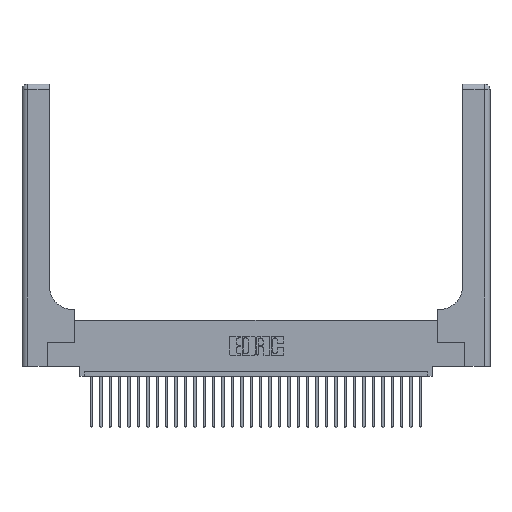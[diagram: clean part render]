
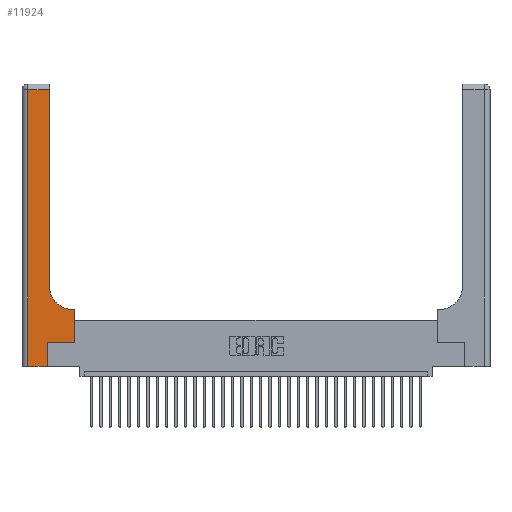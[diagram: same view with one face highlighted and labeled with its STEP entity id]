
A CAD part, top view. The second image highlights one B-rep face of the part: STEP entity #11924.
In plain terms, the highlighted planar face has unit normal (0, 0, 1).
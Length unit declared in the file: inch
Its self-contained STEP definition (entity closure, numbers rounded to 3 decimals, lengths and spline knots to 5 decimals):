
#829 = DIRECTION ( 'NONE',  ( 1., 0., 0. ) ) ;
#990 = EDGE_CURVE ( 'NONE', #28416, #30081, #33058, .T. ) ;
#1725 = VERTEX_POINT ( 'NONE', #17095 ) ;
#1779 = FACE_OUTER_BOUND ( 'NONE', #15088, .T. ) ;
#1963 = CARTESIAN_POINT ( 'NONE',  ( 0.06, 0., 0.37 ) ) ;
#2214 = CARTESIAN_POINT ( 'NONE',  ( 0.5415, 0.6, 0.37 ) ) ;
#3180 = DIRECTION ( 'NONE',  ( 0., 0., -1. ) ) ;
#3660 = EDGE_CURVE ( 'NONE', #8271, #12880, #32105, .T. ) ;
#3897 = PLANE ( 'NONE',  #26352 ) ;
#4772 = VECTOR ( 'NONE', #16548, 39.37008 ) ;
#4850 = ORIENTED_EDGE ( 'NONE', *, *, #29802, .T. ) ;
#6014 = LINE ( 'NONE', #14573, #11296 ) ;
#6174 = DIRECTION ( 'NONE',  ( -1., 0., 0. ) ) ;
#7268 = VECTOR ( 'NONE', #19096, 39.37008 ) ;
#7800 = VECTOR ( 'NONE', #6174, 39.37008 ) ;
#7850 = CARTESIAN_POINT ( 'NONE',  ( 0.5415, 0.85, 0.37 ) ) ;
#8129 = VECTOR ( 'NONE', #28614, 39.37008 ) ;
#8271 = VERTEX_POINT ( 'NONE', #2214 ) ;
#8856 = LINE ( 'NONE', #20960, #11281 ) ;
#9291 = ORIENTED_EDGE ( 'NONE', *, *, #30103, .T. ) ;
#9566 = CARTESIAN_POINT ( 'NONE',  ( 0.5585, 0.6, 0.37 ) ) ;
#9749 = ORIENTED_EDGE ( 'NONE', *, *, #14165, .T. ) ;
#10000 = CARTESIAN_POINT ( 'NONE',  ( 0.2915, 2.94, 0.37 ) ) ;
#10071 = ORIENTED_EDGE ( 'NONE', *, *, #16165, .T. ) ;
#10427 = ORIENTED_EDGE ( 'NONE', *, *, #990, .T. ) ;
#10534 = ORIENTED_EDGE ( 'NONE', *, *, #3660, .T. ) ;
#10969 = DIRECTION ( 'NONE',  ( 0., 1., 0. ) ) ;
#11235 = CARTESIAN_POINT ( 'NONE',  ( 0.2915, 3., 0.37 ) ) ;
#11281 = VECTOR ( 'NONE', #10969, 39.37008 ) ;
#11296 = VECTOR ( 'NONE', #32363, 39.37008 ) ;
#11427 = VERTEX_POINT ( 'NONE', #26280 ) ;
#11924 = ADVANCED_FACE ( 'NONE', ( #1779 ), #3897, .F. ) ;
#12660 = LINE ( 'NONE', #14580, #21778 ) ;
#12880 = VERTEX_POINT ( 'NONE', #15978 ) ;
#13284 = LINE ( 'NONE', #11235, #7268 ) ;
#13596 = CARTESIAN_POINT ( 'NONE',  ( 0.5585, 0.25, 0.37 ) ) ;
#13785 = LINE ( 'NONE', #18516, #8129 ) ;
#14165 = EDGE_CURVE ( 'NONE', #12880, #28416, #13284, .T. ) ;
#14573 = CARTESIAN_POINT ( 'NONE',  ( 0., 0., 0.37 ) ) ;
#14580 = CARTESIAN_POINT ( 'NONE',  ( 0.5585, 0.25, 0.37 ) ) ;
#15088 = EDGE_LOOP ( 'NONE', ( #9749, #10427, #16967, #4850, #9291, #10071, #16710, #17479, #10534 ) ) ;
#15978 = CARTESIAN_POINT ( 'NONE',  ( 0.2915, 0.85, 0.37 ) ) ;
#16165 = EDGE_CURVE ( 'NONE', #1725, #28054, #31559, .T. ) ;
#16548 = DIRECTION ( 'NONE',  ( -1., 0., 0. ) ) ;
#16710 = ORIENTED_EDGE ( 'NONE', *, *, #31509, .T. ) ;
#16967 = ORIENTED_EDGE ( 'NONE', *, *, #28578, .T. ) ;
#17095 = CARTESIAN_POINT ( 'NONE',  ( 0.269, 0.25, 0.37 ) ) ;
#17479 = ORIENTED_EDGE ( 'NONE', *, *, #30250, .T. ) ;
#18516 = CARTESIAN_POINT ( 'NONE',  ( 0.06, 3., 0.37 ) ) ;
#19096 = DIRECTION ( 'NONE',  ( 0., 1., 0. ) ) ;
#19839 = DIRECTION ( 'NONE',  ( 1., 0., 0. ) ) ;
#20217 = CARTESIAN_POINT ( 'NONE',  ( 0.06, 2.94, 0.37 ) ) ;
#20960 = CARTESIAN_POINT ( 'NONE',  ( 0.269, 0., 0.37 ) ) ;
#21778 = VECTOR ( 'NONE', #24830, 39.37008 ) ;
#22299 = VECTOR ( 'NONE', #19839, 39.37008 ) ;
#23498 = CARTESIAN_POINT ( 'NONE',  ( 0., 2.94, 0.37 ) ) ;
#24050 = CARTESIAN_POINT ( 'NONE',  ( 0., 3., 0.37 ) ) ;
#24830 = DIRECTION ( 'NONE',  ( 0., 1., 0. ) ) ;
#26263 = VERTEX_POINT ( 'NONE', #9566 ) ;
#26280 = CARTESIAN_POINT ( 'NONE',  ( 0.269, 0., 0.37 ) ) ;
#26352 = AXIS2_PLACEMENT_3D ( 'NONE', #24050, #31938, #26743 ) ;
#26743 = DIRECTION ( 'NONE',  ( -1., 0., 0. ) ) ;
#27131 = CARTESIAN_POINT ( 'NONE',  ( 0.269, 0.25, 0.37 ) ) ;
#27643 = LINE ( 'NONE', #29279, #4772 ) ;
#28054 = VERTEX_POINT ( 'NONE', #13596 ) ;
#28416 = VERTEX_POINT ( 'NONE', #10000 ) ;
#28578 = EDGE_CURVE ( 'NONE', #30081, #32816, #13785, .T. ) ;
#28614 = DIRECTION ( 'NONE',  ( 0., -1., 0. ) ) ;
#29230 = AXIS2_PLACEMENT_3D ( 'NONE', #7850, #3180, #829 ) ;
#29279 = CARTESIAN_POINT ( 'NONE',  ( 0.2915, 0.6, 0.37 ) ) ;
#29802 = EDGE_CURVE ( 'NONE', #32816, #11427, #6014, .T. ) ;
#30081 = VERTEX_POINT ( 'NONE', #20217 ) ;
#30103 = EDGE_CURVE ( 'NONE', #11427, #1725, #8856, .T. ) ;
#30250 = EDGE_CURVE ( 'NONE', #26263, #8271, #27643, .T. ) ;
#31509 = EDGE_CURVE ( 'NONE', #28054, #26263, #12660, .T. ) ;
#31559 = LINE ( 'NONE', #27131, #22299 ) ;
#31938 = DIRECTION ( 'NONE',  ( 0., 0., -1. ) ) ;
#32105 = CIRCLE ( 'NONE', #29230, 0.25 ) ;
#32363 = DIRECTION ( 'NONE',  ( 1., 0., 0. ) ) ;
#32816 = VERTEX_POINT ( 'NONE', #1963 ) ;
#33058 = LINE ( 'NONE', #23498, #7800 ) ;
